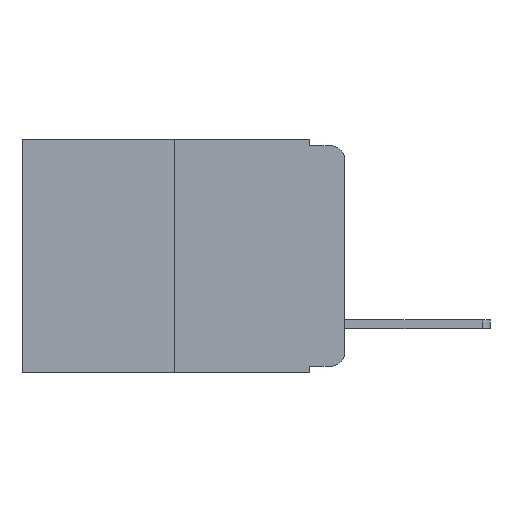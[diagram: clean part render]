
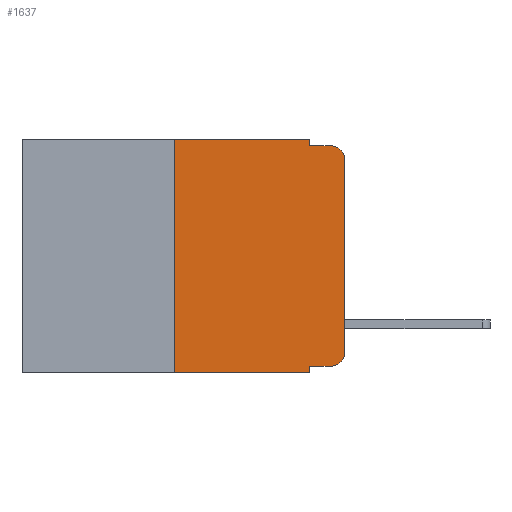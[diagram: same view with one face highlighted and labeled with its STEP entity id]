
A CAD part, left-side view. The second image highlights one B-rep face of the part: STEP entity #1637.
In plain terms, the highlighted planar face has unit normal (-1, 0, 0).
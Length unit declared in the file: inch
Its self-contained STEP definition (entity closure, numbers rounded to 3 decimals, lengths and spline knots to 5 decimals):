
#83 = ORIENTED_EDGE ( 'NONE', *, *, #5854, .T. ) ;
#179 = CARTESIAN_POINT ( 'NONE',  ( 0., 0.02, -0.01 ) ) ;
#217 = ORIENTED_EDGE ( 'NONE', *, *, #7219, .F. ) ;
#300 = ORIENTED_EDGE ( 'NONE', *, *, #6218, .F. ) ;
#385 = EDGE_CURVE ( 'NONE', #5705, #8013, #1827, .T. ) ;
#477 = CARTESIAN_POINT ( 'NONE',  ( 0., 0.02, -0.03 ) ) ;
#503 = DIRECTION ( 'NONE',  ( -1., 0., 0. ) ) ;
#522 = EDGE_CURVE ( 'NONE', #2850, #857, #2743, .T. ) ;
#530 = DIRECTION ( 'NONE',  ( 0., 0., -1. ) ) ;
#575 = ORIENTED_EDGE ( 'NONE', *, *, #7319, .T. ) ;
#620 = DIRECTION ( 'NONE',  ( 0., 0., 1. ) ) ;
#849 = CARTESIAN_POINT ( 'NONE',  ( 0., 0.02, -0.333 ) ) ;
#857 = VERTEX_POINT ( 'NONE', #179 ) ;
#950 = ORIENTED_EDGE ( 'NONE', *, *, #385, .T. ) ;
#958 = CARTESIAN_POINT ( 'NONE',  ( 0., 0.051, 0. ) ) ;
#1261 = DIRECTION ( 'NONE',  ( 0., 0., 1. ) ) ;
#1278 = AXIS2_PLACEMENT_3D ( 'NONE', #10024, #9693, #9718 ) ;
#1434 = DIRECTION ( 'NONE',  ( 0., -1., 0. ) ) ;
#1477 = ORIENTED_EDGE ( 'NONE', *, *, #8739, .F. ) ;
#1544 = VECTOR ( 'NONE', #1434, 39.37008 ) ;
#1637 = ADVANCED_FACE ( 'NONE', ( #9493 ), #5256, .F. ) ;
#1827 = LINE ( 'NONE', #4157, #1544 ) ;
#1880 = VERTEX_POINT ( 'NONE', #3817 ) ;
#2094 = LINE ( 'NONE', #8518, #8306 ) ;
#2414 = CARTESIAN_POINT ( 'NONE',  ( 0., 0.473, 0. ) ) ;
#2743 = LINE ( 'NONE', #7346, #6709 ) ;
#2850 = VERTEX_POINT ( 'NONE', #9536 ) ;
#2916 = VECTOR ( 'NONE', #3460, 39.37008 ) ;
#2928 = ORIENTED_EDGE ( 'NONE', *, *, #9620, .F. ) ;
#3175 = LINE ( 'NONE', #9953, #2916 ) ;
#3300 = EDGE_LOOP ( 'NONE', ( #3593, #3708, #3331, #2928, #1477, #217, #83, #300, #950, #575 ) ) ;
#3331 = ORIENTED_EDGE ( 'NONE', *, *, #522, .F. ) ;
#3460 = DIRECTION ( 'NONE',  ( 0., -1., 0. ) ) ;
#3482 = VERTEX_POINT ( 'NONE', #7243 ) ;
#3521 = CIRCLE ( 'NONE', #1278, 0.02 ) ;
#3593 = ORIENTED_EDGE ( 'NONE', *, *, #7275, .T. ) ;
#3708 = ORIENTED_EDGE ( 'NONE', *, *, #5235, .T. ) ;
#3817 = CARTESIAN_POINT ( 'NONE',  ( 0., 0.25, 0. ) ) ;
#3903 = CARTESIAN_POINT ( 'NONE',  ( 0., 0.051, -0.333 ) ) ;
#4149 = VECTOR ( 'NONE', #4498, 39.37008 ) ;
#4157 = CARTESIAN_POINT ( 'NONE',  ( 0., 0.051, -0.333 ) ) ;
#4195 = VECTOR ( 'NONE', #7858, 39.37008 ) ;
#4264 = VERTEX_POINT ( 'NONE', #7376 ) ;
#4341 = CIRCLE ( 'NONE', #6187, 0.02 ) ;
#4451 = CARTESIAN_POINT ( 'NONE',  ( 0., 0., -0.03 ) ) ;
#4498 = DIRECTION ( 'NONE',  ( 0., 0., -1. ) ) ;
#4844 = CARTESIAN_POINT ( 'NONE',  ( 0., 0.473, 0. ) ) ;
#4983 = CARTESIAN_POINT ( 'NONE',  ( 0., 0.25, 0. ) ) ;
#5235 = EDGE_CURVE ( 'NONE', #7452, #857, #4341, .T. ) ;
#5256 = PLANE ( 'NONE',  #9310 ) ;
#5414 = LINE ( 'NONE', #2414, #9301 ) ;
#5562 = CARTESIAN_POINT ( 'NONE',  ( 0., 0., -0.313 ) ) ;
#5705 = VERTEX_POINT ( 'NONE', #3903 ) ;
#5854 = EDGE_CURVE ( 'NONE', #3482, #4264, #3175, .T. ) ;
#6187 = AXIS2_PLACEMENT_3D ( 'NONE', #477, #503, #530 ) ;
#6218 = EDGE_CURVE ( 'NONE', #5705, #4264, #6288, .T. ) ;
#6288 = LINE ( 'NONE', #8397, #4195 ) ;
#6612 = VECTOR ( 'NONE', #620, 39.37008 ) ;
#6709 = VECTOR ( 'NONE', #7611, 39.37008 ) ;
#7219 = EDGE_CURVE ( 'NONE', #3482, #1880, #8539, .T. ) ;
#7243 = CARTESIAN_POINT ( 'NONE',  ( 0., 0.25, -0.343 ) ) ;
#7275 = EDGE_CURVE ( 'NONE', #7563, #7452, #2094, .T. ) ;
#7319 = EDGE_CURVE ( 'NONE', #8013, #7563, #3521, .T. ) ;
#7346 = CARTESIAN_POINT ( 'NONE',  ( 0., 0.051, -0.01 ) ) ;
#7376 = CARTESIAN_POINT ( 'NONE',  ( 0., 0.051, -0.343 ) ) ;
#7452 = VERTEX_POINT ( 'NONE', #4451 ) ;
#7547 = CARTESIAN_POINT ( 'NONE',  ( 0., 0.051, 0. ) ) ;
#7563 = VERTEX_POINT ( 'NONE', #5562 ) ;
#7611 = DIRECTION ( 'NONE',  ( 0., -1., 0. ) ) ;
#7858 = DIRECTION ( 'NONE',  ( 0., 0., -1. ) ) ;
#7867 = DIRECTION ( 'NONE',  ( 1., 0., 0. ) ) ;
#7884 = DIRECTION ( 'NONE',  ( 0., -1., 0. ) ) ;
#8013 = VERTEX_POINT ( 'NONE', #849 ) ;
#8306 = VECTOR ( 'NONE', #1261, 39.37008 ) ;
#8397 = CARTESIAN_POINT ( 'NONE',  ( 0., 0.051, 0. ) ) ;
#8411 = LINE ( 'NONE', #7547, #4149 ) ;
#8468 = DIRECTION ( 'NONE',  ( 0., 0., -1. ) ) ;
#8518 = CARTESIAN_POINT ( 'NONE',  ( 0., 0., 0. ) ) ;
#8539 = LINE ( 'NONE', #4983, #6612 ) ;
#8739 = EDGE_CURVE ( 'NONE', #1880, #9507, #5414, .T. ) ;
#9301 = VECTOR ( 'NONE', #7884, 39.37008 ) ;
#9310 = AXIS2_PLACEMENT_3D ( 'NONE', #4844, #7867, #8468 ) ;
#9493 = FACE_OUTER_BOUND ( 'NONE', #3300, .T. ) ;
#9507 = VERTEX_POINT ( 'NONE', #958 ) ;
#9536 = CARTESIAN_POINT ( 'NONE',  ( 0., 0.051, -0.01 ) ) ;
#9620 = EDGE_CURVE ( 'NONE', #9507, #2850, #8411, .T. ) ;
#9693 = DIRECTION ( 'NONE',  ( -1., 0., 0. ) ) ;
#9718 = DIRECTION ( 'NONE',  ( 0., 0., -1. ) ) ;
#9953 = CARTESIAN_POINT ( 'NONE',  ( 0., 0.473, -0.343 ) ) ;
#10024 = CARTESIAN_POINT ( 'NONE',  ( 0., 0.02, -0.313 ) ) ;
